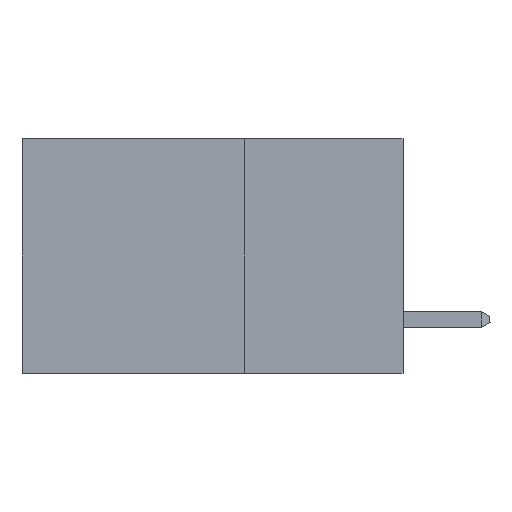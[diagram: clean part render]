
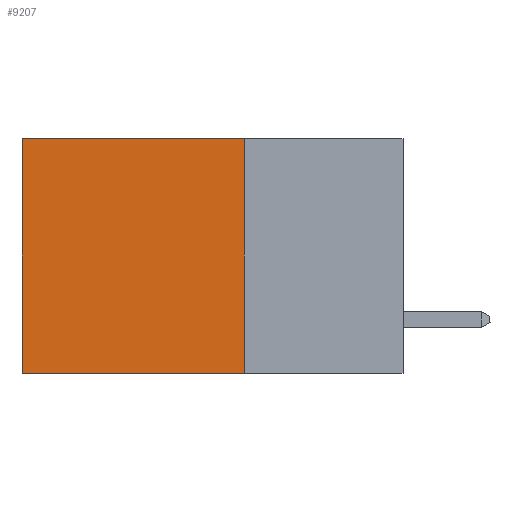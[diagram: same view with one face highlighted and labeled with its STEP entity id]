
A CAD part, left-side view. The second image highlights one B-rep face of the part: STEP entity #9207.
In plain terms, the highlighted planar face has unit normal (-1, 0, 0).
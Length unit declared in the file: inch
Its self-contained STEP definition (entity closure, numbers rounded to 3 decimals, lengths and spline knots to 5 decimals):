
#746 = LINE ( 'NONE', #24546, #4637 ) ;
#1056 = LINE ( 'NONE', #4608, #17839 ) ;
#1774 = VECTOR ( 'NONE', #15526, 39.37008 ) ;
#1906 = DIRECTION ( 'NONE',  ( 0., 1., 0. ) ) ;
#1936 = VECTOR ( 'NONE', #1906, 39.37008 ) ;
#2798 = CARTESIAN_POINT ( 'NONE',  ( 0.2875, 0.6, -0.37 ) ) ;
#4078 = ORIENTED_EDGE ( 'NONE', *, *, #18991, .F. ) ;
#4608 = CARTESIAN_POINT ( 'NONE',  ( 0.2875, 0.25, -0.37 ) ) ;
#4637 = VECTOR ( 'NONE', #22380, 39.37008 ) ;
#4809 = FACE_OUTER_BOUND ( 'NONE', #22645, .T. ) ;
#6591 = DIRECTION ( 'NONE',  ( 0., 0., -1. ) ) ;
#6918 = EDGE_CURVE ( 'NONE', #10013, #18933, #746, .T. ) ;
#7620 = CARTESIAN_POINT ( 'NONE',  ( 0.2875, 0.25, 0. ) ) ;
#7841 = ORIENTED_EDGE ( 'NONE', *, *, #23916, .T. ) ;
#8643 = AXIS2_PLACEMENT_3D ( 'NONE', #24023, #18288, #6591 ) ;
#9207 = ADVANCED_FACE ( 'NONE', ( #4809 ), #21936, .F. ) ;
#10013 = VERTEX_POINT ( 'NONE', #14498 ) ;
#12278 = VERTEX_POINT ( 'NONE', #15034 ) ;
#13036 = EDGE_CURVE ( 'NONE', #20507, #18933, #1056, .T. ) ;
#13220 = CARTESIAN_POINT ( 'NONE',  ( 0.2875, 0.25, -0.37 ) ) ;
#14498 = CARTESIAN_POINT ( 'NONE',  ( 0.2875, 0.6, 0. ) ) ;
#15034 = CARTESIAN_POINT ( 'NONE',  ( 0.2875, 0.25, 0. ) ) ;
#15526 = DIRECTION ( 'NONE',  ( 0., 0., -1. ) ) ;
#17839 = VECTOR ( 'NONE', #18058, 39.37008 ) ;
#18058 = DIRECTION ( 'NONE',  ( 0., 1., 0. ) ) ;
#18288 = DIRECTION ( 'NONE',  ( 1., 0., 0. ) ) ;
#18614 = LINE ( 'NONE', #23441, #1774 ) ;
#18933 = VERTEX_POINT ( 'NONE', #2798 ) ;
#18991 = EDGE_CURVE ( 'NONE', #12278, #20507, #18614, .T. ) ;
#20378 = ORIENTED_EDGE ( 'NONE', *, *, #13036, .F. ) ;
#20507 = VERTEX_POINT ( 'NONE', #13220 ) ;
#21452 = LINE ( 'NONE', #7620, #1936 ) ;
#21936 = PLANE ( 'NONE',  #8643 ) ;
#22007 = ORIENTED_EDGE ( 'NONE', *, *, #6918, .T. ) ;
#22380 = DIRECTION ( 'NONE',  ( 0., 0., -1. ) ) ;
#22645 = EDGE_LOOP ( 'NONE', ( #22007, #20378, #4078, #7841 ) ) ;
#23441 = CARTESIAN_POINT ( 'NONE',  ( 0.2875, 0.25, 0. ) ) ;
#23916 = EDGE_CURVE ( 'NONE', #12278, #10013, #21452, .T. ) ;
#24023 = CARTESIAN_POINT ( 'NONE',  ( 0.2875, 0.25, 0. ) ) ;
#24546 = CARTESIAN_POINT ( 'NONE',  ( 0.2875, 0.6, 0. ) ) ;
